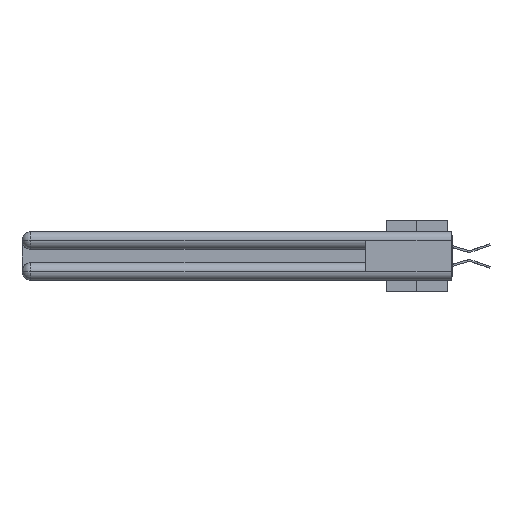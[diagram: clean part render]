
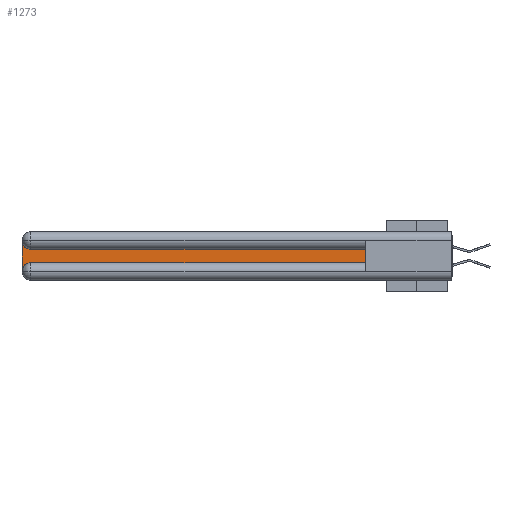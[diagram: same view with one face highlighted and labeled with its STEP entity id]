
A CAD part, left-side view. The second image highlights one B-rep face of the part: STEP entity #1273.
In plain terms, the highlighted planar face has unit normal (-1, 0, 0).
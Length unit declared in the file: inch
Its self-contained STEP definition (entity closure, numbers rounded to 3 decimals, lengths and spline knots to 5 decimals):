
#1052 = VERTEX_POINT ( 'NONE', #3193 ) ;
#1273 = ADVANCED_FACE ( 'NONE', ( #19597 ), #1883, .F. ) ;
#1883 = PLANE ( 'NONE',  #6775 ) ;
#3193 = CARTESIAN_POINT ( 'NONE',  ( 0.075, 2.94, -0.2175 ) ) ;
#4129 = LINE ( 'NONE', #5599, #14190 ) ;
#5168 = VECTOR ( 'NONE', #18750, 39.37008 ) ;
#5599 = CARTESIAN_POINT ( 'NONE',  ( 0.075, 0.6, -0.2175 ) ) ;
#5677 = DIRECTION ( 'NONE',  ( 0., 1., 0. ) ) ;
#6775 = AXIS2_PLACEMENT_3D ( 'NONE', #10225, #27079, #27317 ) ;
#6907 = DIRECTION ( 'NONE',  ( 0., -1., 0. ) ) ;
#7004 = DIRECTION ( 'NONE',  ( 0., 0., -1. ) ) ;
#7157 = EDGE_CURVE ( 'NONE', #1052, #29825, #31421, .T. ) ;
#7705 = LINE ( 'NONE', #11316, #23448 ) ;
#8405 = DIRECTION ( 'NONE',  ( 0., 0., -1. ) ) ;
#8508 = CIRCLE ( 'NONE', #31677, 0.06 ) ;
#9585 = VECTOR ( 'NONE', #6907, 39.37008 ) ;
#9751 = CARTESIAN_POINT ( 'NONE',  ( 0.075, 0.6, -0.2175 ) ) ;
#10225 = CARTESIAN_POINT ( 'NONE',  ( 0.075, 3., -0.1225 ) ) ;
#11316 = CARTESIAN_POINT ( 'NONE',  ( 0.075, 0.6, -0.1225 ) ) ;
#11334 = DIRECTION ( 'NONE',  ( 1., 0., 0. ) ) ;
#13148 = ORIENTED_EDGE ( 'NONE', *, *, #7157, .T. ) ;
#13607 = EDGE_CURVE ( 'NONE', #34001, #1052, #8508, .T. ) ;
#14190 = VECTOR ( 'NONE', #25156, 39.37008 ) ;
#16096 = AXIS2_PLACEMENT_3D ( 'NONE', #18234, #20939, #7004 ) ;
#16146 = ORIENTED_EDGE ( 'NONE', *, *, #27641, .T. ) ;
#18234 = CARTESIAN_POINT ( 'NONE',  ( 0.075, 2.94, -0.0625 ) ) ;
#18732 = LINE ( 'NONE', #35516, #5168 ) ;
#18750 = DIRECTION ( 'NONE',  ( 0., 0., -1. ) ) ;
#19597 = FACE_OUTER_BOUND ( 'NONE', #23649, .T. ) ;
#20452 = ORIENTED_EDGE ( 'NONE', *, *, #33952, .T. ) ;
#20939 = DIRECTION ( 'NONE',  ( 1., 0., 0. ) ) ;
#22334 = CARTESIAN_POINT ( 'NONE',  ( 0.075, 2.94, -0.2775 ) ) ;
#23448 = VECTOR ( 'NONE', #5677, 39.37008 ) ;
#23649 = EDGE_LOOP ( 'NONE', ( #16146, #34759, #36187, #25896, #13148, #20452 ) ) ;
#25156 = DIRECTION ( 'NONE',  ( 0., 0., 1. ) ) ;
#25896 = ORIENTED_EDGE ( 'NONE', *, *, #13607, .T. ) ;
#26157 = CIRCLE ( 'NONE', #16096, 0.06 ) ;
#26231 = EDGE_CURVE ( 'NONE', #31981, #34001, #18732, .T. ) ;
#27079 = DIRECTION ( 'NONE',  ( 1., 0., 0. ) ) ;
#27317 = DIRECTION ( 'NONE',  ( 0., 0., -1. ) ) ;
#27397 = VERTEX_POINT ( 'NONE', #27710 ) ;
#27641 = EDGE_CURVE ( 'NONE', #31042, #27397, #7705, .T. ) ;
#27710 = CARTESIAN_POINT ( 'NONE',  ( 0.075, 2.94, -0.1225 ) ) ;
#29825 = VERTEX_POINT ( 'NONE', #31444 ) ;
#31042 = VERTEX_POINT ( 'NONE', #35283 ) ;
#31189 = EDGE_CURVE ( 'NONE', #27397, #31981, #26157, .T. ) ;
#31421 = LINE ( 'NONE', #9751, #9585 ) ;
#31444 = CARTESIAN_POINT ( 'NONE',  ( 0.075, 0.6, -0.2175 ) ) ;
#31677 = AXIS2_PLACEMENT_3D ( 'NONE', #22334, #11334, #8405 ) ;
#31981 = VERTEX_POINT ( 'NONE', #33710 ) ;
#33710 = CARTESIAN_POINT ( 'NONE',  ( 0.075, 3., -0.0625 ) ) ;
#33952 = EDGE_CURVE ( 'NONE', #29825, #31042, #4129, .T. ) ;
#34001 = VERTEX_POINT ( 'NONE', #34176 ) ;
#34176 = CARTESIAN_POINT ( 'NONE',  ( 0.075, 3., -0.2775 ) ) ;
#34759 = ORIENTED_EDGE ( 'NONE', *, *, #31189, .T. ) ;
#35283 = CARTESIAN_POINT ( 'NONE',  ( 0.075, 0.6, -0.1225 ) ) ;
#35516 = CARTESIAN_POINT ( 'NONE',  ( 0.075, 3., -0.2175 ) ) ;
#36187 = ORIENTED_EDGE ( 'NONE', *, *, #26231, .T. ) ;
